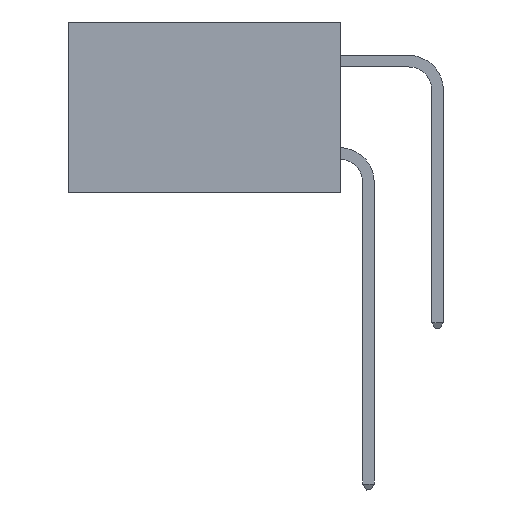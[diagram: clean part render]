
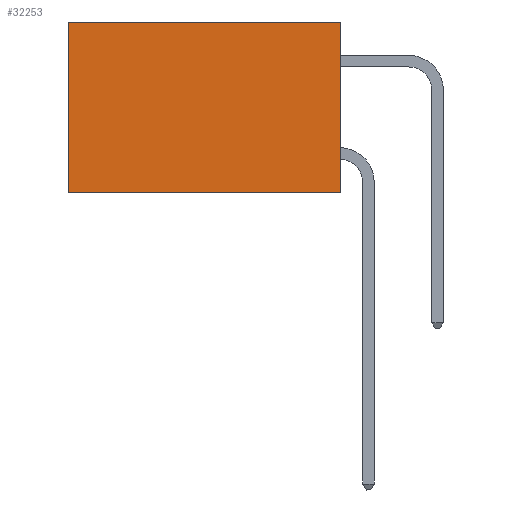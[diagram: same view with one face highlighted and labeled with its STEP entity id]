
A CAD part, left-side view. The second image highlights one B-rep face of the part: STEP entity #32253.
In plain terms, the highlighted planar face has unit normal (-1, 0, 0).
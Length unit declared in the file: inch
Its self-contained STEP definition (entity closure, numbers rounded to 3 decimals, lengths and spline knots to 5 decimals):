
#3216 = ORIENTED_EDGE ( 'NONE', *, *, #28470, .T. ) ;
#3506 = DIRECTION ( 'NONE',  ( 0., 0., -1. ) ) ;
#3652 = VERTEX_POINT ( 'NONE', #22330 ) ;
#4160 = CARTESIAN_POINT ( 'NONE',  ( 0.277, 0., 0. ) ) ;
#4960 = VECTOR ( 'NONE', #3506, 39.37008 ) ;
#6976 = DIRECTION ( 'NONE',  ( 1., 0., 0. ) ) ;
#7752 = VECTOR ( 'NONE', #9687, 39.37008 ) ;
#9687 = DIRECTION ( 'NONE',  ( 0., 1., 0. ) ) ;
#11135 = EDGE_CURVE ( 'NONE', #15539, #3652, #22157, .T. ) ;
#11707 = VECTOR ( 'NONE', #12004, 39.37008 ) ;
#12004 = DIRECTION ( 'NONE',  ( 0., 0., -1. ) ) ;
#12279 = LINE ( 'NONE', #25506, #4960 ) ;
#13479 = AXIS2_PLACEMENT_3D ( 'NONE', #20752, #6976, #26385 ) ;
#14742 = VECTOR ( 'NONE', #21880, 39.37008 ) ;
#14939 = PLANE ( 'NONE',  #13479 ) ;
#15539 = VERTEX_POINT ( 'NONE', #27059 ) ;
#16448 = FACE_OUTER_BOUND ( 'NONE', #28952, .T. ) ;
#17387 = ORIENTED_EDGE ( 'NONE', *, *, #32770, .F. ) ;
#20752 = CARTESIAN_POINT ( 'NONE',  ( 0.277, 0., -0.37 ) ) ;
#21761 = CARTESIAN_POINT ( 'NONE',  ( 0.277, 0., -0.37 ) ) ;
#21880 = DIRECTION ( 'NONE',  ( 0., 1., 0. ) ) ;
#22157 = LINE ( 'NONE', #21761, #14742 ) ;
#22330 = CARTESIAN_POINT ( 'NONE',  ( 0.277, 0.59, -0.37 ) ) ;
#22679 = VERTEX_POINT ( 'NONE', #34130 ) ;
#25255 = ORIENTED_EDGE ( 'NONE', *, *, #11135, .F. ) ;
#25506 = CARTESIAN_POINT ( 'NONE',  ( 0.277, 0.59, -0.37 ) ) ;
#26385 = DIRECTION ( 'NONE',  ( 0., 0., -1. ) ) ;
#26496 = LINE ( 'NONE', #34020, #11707 ) ;
#27059 = CARTESIAN_POINT ( 'NONE',  ( 0.277, 0., -0.37 ) ) ;
#27163 = ORIENTED_EDGE ( 'NONE', *, *, #33673, .T. ) ;
#28470 = EDGE_CURVE ( 'NONE', #22679, #3652, #12279, .T. ) ;
#28952 = EDGE_LOOP ( 'NONE', ( #3216, #25255, #17387, #27163 ) ) ;
#29829 = LINE ( 'NONE', #4160, #7752 ) ;
#31568 = VERTEX_POINT ( 'NONE', #34580 ) ;
#32253 = ADVANCED_FACE ( 'NONE', ( #16448 ), #14939, .F. ) ;
#32770 = EDGE_CURVE ( 'NONE', #31568, #15539, #26496, .T. ) ;
#33673 = EDGE_CURVE ( 'NONE', #31568, #22679, #29829, .T. ) ;
#34020 = CARTESIAN_POINT ( 'NONE',  ( 0.277, 0., -0.37 ) ) ;
#34130 = CARTESIAN_POINT ( 'NONE',  ( 0.277, 0.59, 0. ) ) ;
#34580 = CARTESIAN_POINT ( 'NONE',  ( 0.277, 0., 0. ) ) ;
